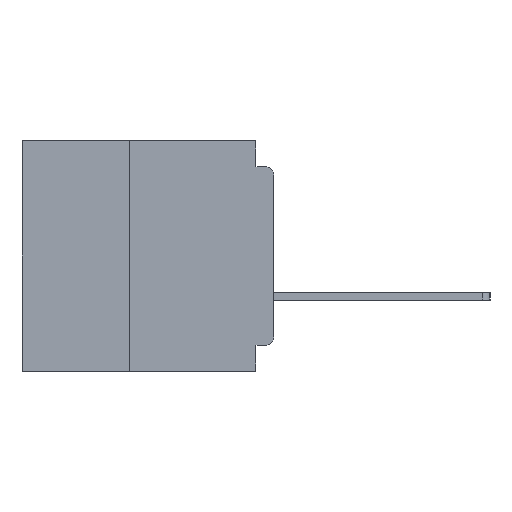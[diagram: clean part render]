
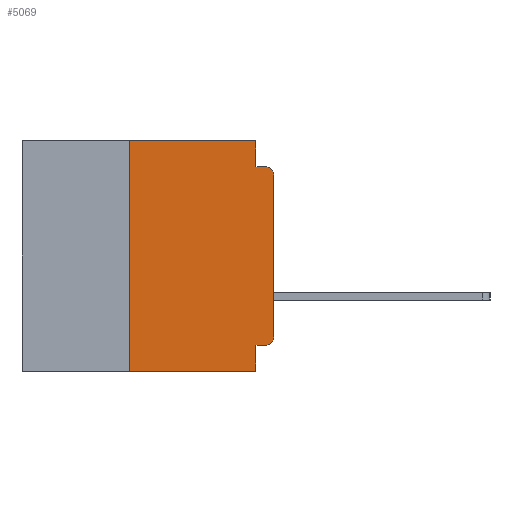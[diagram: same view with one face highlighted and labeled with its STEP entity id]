
A CAD part, left-side view. The second image highlights one B-rep face of the part: STEP entity #5069.
In plain terms, the highlighted planar face has unit normal (-1, 0, 0).
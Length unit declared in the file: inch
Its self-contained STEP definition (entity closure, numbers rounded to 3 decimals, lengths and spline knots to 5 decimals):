
#4 = VECTOR ( 'NONE', #16149, 39.37008 ) ;
#733 = ORIENTED_EDGE ( 'NONE', *, *, #36994, .T. ) ;
#1969 = CARTESIAN_POINT ( 'NONE',  ( 0., 0.031, 0. ) ) ;
#2126 = EDGE_CURVE ( 'NONE', #31939, #18100, #5633, .T. ) ;
#2263 = VERTEX_POINT ( 'NONE', #17335 ) ;
#2988 = ORIENTED_EDGE ( 'NONE', *, *, #33958, .T. ) ;
#3307 = CARTESIAN_POINT ( 'NONE',  ( 0., 0., -0.355 ) ) ;
#3798 = VERTEX_POINT ( 'NONE', #36937 ) ;
#3870 = CARTESIAN_POINT ( 'NONE',  ( 0., 0.031, -0.045 ) ) ;
#4559 = CARTESIAN_POINT ( 'NONE',  ( 0., 0.437, 0. ) ) ;
#4635 = ORIENTED_EDGE ( 'NONE', *, *, #18082, .F. ) ;
#5069 = ADVANCED_FACE ( 'NONE', ( #26568 ), #31766, .F. ) ;
#5298 = EDGE_LOOP ( 'NONE', ( #22544, #17044, #4635, #31461, #23848, #24810, #733, #30597, #10777, #2988 ) ) ;
#5590 = VECTOR ( 'NONE', #24620, 39.37008 ) ;
#5633 = LINE ( 'NONE', #1969, #13518 ) ;
#6718 = CARTESIAN_POINT ( 'NONE',  ( 0., 0., -0.045 ) ) ;
#6728 = EDGE_CURVE ( 'NONE', #33645, #3798, #7440, .T. ) ;
#6878 = CARTESIAN_POINT ( 'NONE',  ( 0., 0.031, -0.4 ) ) ;
#7254 = DIRECTION ( 'NONE',  ( 0., -1., 0. ) ) ;
#7346 = CARTESIAN_POINT ( 'NONE',  ( 0., 0.015, -0.06 ) ) ;
#7440 = LINE ( 'NONE', #6878, #5590 ) ;
#7464 = EDGE_CURVE ( 'NONE', #2263, #15259, #10163, .T. ) ;
#7842 = LINE ( 'NONE', #19060, #4 ) ;
#10163 = CIRCLE ( 'NONE', #19529, 0.015 ) ;
#10306 = LINE ( 'NONE', #6718, #32835 ) ;
#10333 = DIRECTION ( 'NONE',  ( 0., 0., -1. ) ) ;
#10777 = ORIENTED_EDGE ( 'NONE', *, *, #30120, .F. ) ;
#11126 = VERTEX_POINT ( 'NONE', #29723 ) ;
#11664 = DIRECTION ( 'NONE',  ( -1., 0., 0. ) ) ;
#12117 = DIRECTION ( 'NONE',  ( 0., 1., 0. ) ) ;
#12383 = DIRECTION ( 'NONE',  ( 0., -1., 0. ) ) ;
#12523 = VERTEX_POINT ( 'NONE', #17781 ) ;
#13222 = EDGE_CURVE ( 'NONE', #12523, #31939, #23048, .T. ) ;
#13518 = VECTOR ( 'NONE', #38146, 39.37008 ) ;
#14146 = DIRECTION ( 'NONE',  ( 1., 0., 0. ) ) ;
#15259 = VERTEX_POINT ( 'NONE', #27390 ) ;
#15592 = LINE ( 'NONE', #16483, #23498 ) ;
#16149 = DIRECTION ( 'NONE',  ( 0., 0., 1. ) ) ;
#16483 = CARTESIAN_POINT ( 'NONE',  ( 0., 0., 0. ) ) ;
#17044 = ORIENTED_EDGE ( 'NONE', *, *, #7464, .T. ) ;
#17335 = CARTESIAN_POINT ( 'NONE',  ( 0., 0., -0.06 ) ) ;
#17781 = CARTESIAN_POINT ( 'NONE',  ( 0., 0.25, 0. ) ) ;
#17982 = CIRCLE ( 'NONE', #36572, 0.015 ) ;
#18082 = EDGE_CURVE ( 'NONE', #18100, #15259, #10306, .T. ) ;
#18100 = VERTEX_POINT ( 'NONE', #3870 ) ;
#18375 = CARTESIAN_POINT ( 'NONE',  ( 0., 0.437, 0. ) ) ;
#18791 = LINE ( 'NONE', #3307, #19723 ) ;
#19060 = CARTESIAN_POINT ( 'NONE',  ( 0., 0.25, -0.4 ) ) ;
#19475 = AXIS2_PLACEMENT_3D ( 'NONE', #4559, #14146, #34690 ) ;
#19479 = DIRECTION ( 'NONE',  ( 0., 0., 1. ) ) ;
#19529 = AXIS2_PLACEMENT_3D ( 'NONE', #7346, #28011, #10333 ) ;
#19723 = VECTOR ( 'NONE', #12117, 39.37008 ) ;
#20102 = CARTESIAN_POINT ( 'NONE',  ( 0., 0., -0.34 ) ) ;
#20220 = VERTEX_POINT ( 'NONE', #20102 ) ;
#21486 = DIRECTION ( 'NONE',  ( 0., -1., 0. ) ) ;
#22544 = ORIENTED_EDGE ( 'NONE', *, *, #29146, .T. ) ;
#23048 = LINE ( 'NONE', #18375, #37631 ) ;
#23498 = VECTOR ( 'NONE', #19479, 39.37008 ) ;
#23848 = ORIENTED_EDGE ( 'NONE', *, *, #13222, .F. ) ;
#24620 = DIRECTION ( 'NONE',  ( 0., 0., -1. ) ) ;
#24810 = ORIENTED_EDGE ( 'NONE', *, *, #32505, .F. ) ;
#24848 = CARTESIAN_POINT ( 'NONE',  ( 0., 0.437, -0.4 ) ) ;
#25005 = CARTESIAN_POINT ( 'NONE',  ( 0., 0.031, -0.355 ) ) ;
#25137 = CARTESIAN_POINT ( 'NONE',  ( 0., 0.031, 0. ) ) ;
#25694 = VERTEX_POINT ( 'NONE', #36262 ) ;
#26568 = FACE_OUTER_BOUND ( 'NONE', #5298, .T. ) ;
#26985 = VECTOR ( 'NONE', #7254, 39.37008 ) ;
#27390 = CARTESIAN_POINT ( 'NONE',  ( 0., 0.015, -0.045 ) ) ;
#28011 = DIRECTION ( 'NONE',  ( -1., 0., 0. ) ) ;
#29146 = EDGE_CURVE ( 'NONE', #20220, #2263, #15592, .T. ) ;
#29320 = CARTESIAN_POINT ( 'NONE',  ( 0., 0.015, -0.34 ) ) ;
#29723 = CARTESIAN_POINT ( 'NONE',  ( 0., 0.25, -0.4 ) ) ;
#30120 = EDGE_CURVE ( 'NONE', #25694, #33645, #18791, .T. ) ;
#30597 = ORIENTED_EDGE ( 'NONE', *, *, #6728, .F. ) ;
#31461 = ORIENTED_EDGE ( 'NONE', *, *, #2126, .F. ) ;
#31766 = PLANE ( 'NONE',  #19475 ) ;
#31939 = VERTEX_POINT ( 'NONE', #25137 ) ;
#32239 = DIRECTION ( 'NONE',  ( 0., 0., -1. ) ) ;
#32505 = EDGE_CURVE ( 'NONE', #11126, #12523, #7842, .T. ) ;
#32835 = VECTOR ( 'NONE', #21486, 39.37008 ) ;
#33645 = VERTEX_POINT ( 'NONE', #25005 ) ;
#33958 = EDGE_CURVE ( 'NONE', #25694, #20220, #17982, .T. ) ;
#34690 = DIRECTION ( 'NONE',  ( 0., 0., -1. ) ) ;
#36262 = CARTESIAN_POINT ( 'NONE',  ( 0., 0.015, -0.355 ) ) ;
#36527 = LINE ( 'NONE', #24848, #26985 ) ;
#36572 = AXIS2_PLACEMENT_3D ( 'NONE', #29320, #11664, #32239 ) ;
#36937 = CARTESIAN_POINT ( 'NONE',  ( 0., 0.031, -0.4 ) ) ;
#36994 = EDGE_CURVE ( 'NONE', #11126, #3798, #36527, .T. ) ;
#37631 = VECTOR ( 'NONE', #12383, 39.37008 ) ;
#38146 = DIRECTION ( 'NONE',  ( 0., 0., -1. ) ) ;
